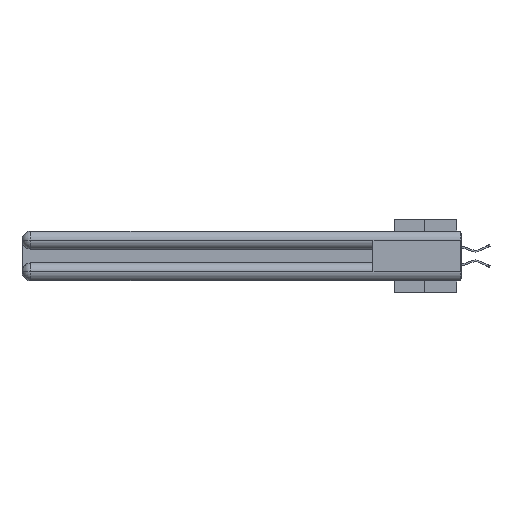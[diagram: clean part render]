
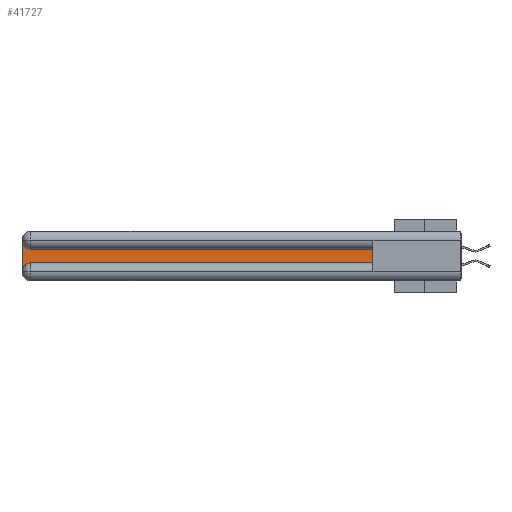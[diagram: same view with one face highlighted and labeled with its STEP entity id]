
A CAD part, left-side view. The second image highlights one B-rep face of the part: STEP entity #41727.
In plain terms, the highlighted planar face has unit normal (-1, 0, 0).
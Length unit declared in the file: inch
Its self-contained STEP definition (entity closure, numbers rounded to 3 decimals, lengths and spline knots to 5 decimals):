
#301 = VERTEX_POINT ( 'NONE', #36334 ) ;
#541 = AXIS2_PLACEMENT_3D ( 'NONE', #25504, #21636, #22047 ) ;
#859 = CARTESIAN_POINT ( 'NONE',  ( 0.075, 2.94, -0.2775 ) ) ;
#1934 = CARTESIAN_POINT ( 'NONE',  ( 0.075, 0.6, -0.1225 ) ) ;
#3647 = EDGE_CURVE ( 'NONE', #40863, #16322, #29112, .T. ) ;
#3972 = ORIENTED_EDGE ( 'NONE', *, *, #11105, .T. ) ;
#4729 = DIRECTION ( 'NONE',  ( 0., 0., -1. ) ) ;
#5155 = CARTESIAN_POINT ( 'NONE',  ( 0.075, 3., -0.2175 ) ) ;
#5237 = DIRECTION ( 'NONE',  ( 0., 1., 0. ) ) ;
#5782 = DIRECTION ( 'NONE',  ( 1., 0., 0. ) ) ;
#7307 = DIRECTION ( 'NONE',  ( 0., 0., -1. ) ) ;
#7338 = VECTOR ( 'NONE', #8564, 39.37008 ) ;
#8532 = VECTOR ( 'NONE', #16157, 39.37008 ) ;
#8564 = DIRECTION ( 'NONE',  ( 0., 0., 1. ) ) ;
#9381 = CARTESIAN_POINT ( 'NONE',  ( 0.075, 0.6, -0.2175 ) ) ;
#10780 = VECTOR ( 'NONE', #5237, 39.37008 ) ;
#10840 = VERTEX_POINT ( 'NONE', #12940 ) ;
#11105 = EDGE_CURVE ( 'NONE', #15777, #10840, #13010, .T. ) ;
#12940 = CARTESIAN_POINT ( 'NONE',  ( 0.075, 0.6, -0.1225 ) ) ;
#13010 = LINE ( 'NONE', #24944, #7338 ) ;
#14233 = CIRCLE ( 'NONE', #31310, 0.06 ) ;
#15691 = EDGE_CURVE ( 'NONE', #16322, #42366, #14233, .T. ) ;
#15777 = VERTEX_POINT ( 'NONE', #37459 ) ;
#16157 = DIRECTION ( 'NONE',  ( 0., -1., 0. ) ) ;
#16322 = VERTEX_POINT ( 'NONE', #24055 ) ;
#19557 = LINE ( 'NONE', #1934, #10780 ) ;
#20577 = EDGE_CURVE ( 'NONE', #10840, #301, #19557, .T. ) ;
#20977 = LINE ( 'NONE', #9381, #8532 ) ;
#21636 = DIRECTION ( 'NONE',  ( 1., 0., 0. ) ) ;
#22047 = DIRECTION ( 'NONE',  ( 0., 0., -1. ) ) ;
#22050 = PLANE ( 'NONE',  #26077 ) ;
#24055 = CARTESIAN_POINT ( 'NONE',  ( 0.075, 3., -0.2775 ) ) ;
#24944 = CARTESIAN_POINT ( 'NONE',  ( 0.075, 0.6, -0.2175 ) ) ;
#25086 = ORIENTED_EDGE ( 'NONE', *, *, #3647, .T. ) ;
#25504 = CARTESIAN_POINT ( 'NONE',  ( 0.075, 2.94, -0.0625 ) ) ;
#25645 = CARTESIAN_POINT ( 'NONE',  ( 0.075, 3., -0.1225 ) ) ;
#26077 = AXIS2_PLACEMENT_3D ( 'NONE', #25645, #5782, #35249 ) ;
#27683 = ORIENTED_EDGE ( 'NONE', *, *, #15691, .T. ) ;
#27901 = ORIENTED_EDGE ( 'NONE', *, *, #20577, .T. ) ;
#28603 = ORIENTED_EDGE ( 'NONE', *, *, #30292, .T. ) ;
#29112 = LINE ( 'NONE', #5155, #35729 ) ;
#30292 = EDGE_CURVE ( 'NONE', #42366, #15777, #20977, .T. ) ;
#31310 = AXIS2_PLACEMENT_3D ( 'NONE', #859, #40051, #7307 ) ;
#32205 = EDGE_CURVE ( 'NONE', #301, #40863, #33766, .T. ) ;
#32332 = ORIENTED_EDGE ( 'NONE', *, *, #32205, .T. ) ;
#33766 = CIRCLE ( 'NONE', #541, 0.06 ) ;
#34194 = FACE_OUTER_BOUND ( 'NONE', #39341, .T. ) ;
#35157 = CARTESIAN_POINT ( 'NONE',  ( 0.075, 3., -0.0625 ) ) ;
#35249 = DIRECTION ( 'NONE',  ( 0., 0., -1. ) ) ;
#35342 = CARTESIAN_POINT ( 'NONE',  ( 0.075, 2.94, -0.2175 ) ) ;
#35729 = VECTOR ( 'NONE', #4729, 39.37008 ) ;
#36334 = CARTESIAN_POINT ( 'NONE',  ( 0.075, 2.94, -0.1225 ) ) ;
#37459 = CARTESIAN_POINT ( 'NONE',  ( 0.075, 0.6, -0.2175 ) ) ;
#39341 = EDGE_LOOP ( 'NONE', ( #27901, #32332, #25086, #27683, #28603, #3972 ) ) ;
#40051 = DIRECTION ( 'NONE',  ( 1., 0., 0. ) ) ;
#40863 = VERTEX_POINT ( 'NONE', #35157 ) ;
#41727 = ADVANCED_FACE ( 'NONE', ( #34194 ), #22050, .F. ) ;
#42366 = VERTEX_POINT ( 'NONE', #35342 ) ;
